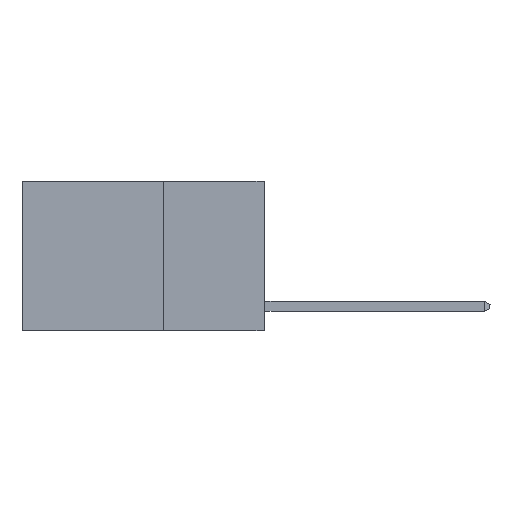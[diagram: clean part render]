
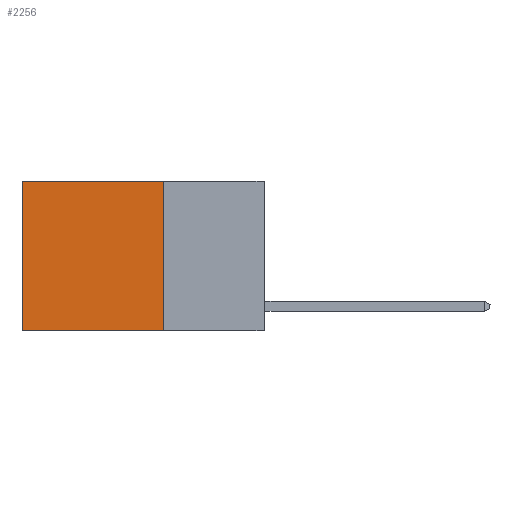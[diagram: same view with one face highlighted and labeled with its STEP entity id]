
A CAD part, left-side view. The second image highlights one B-rep face of the part: STEP entity #2256.
In plain terms, the highlighted planar face has unit normal (-1, 0, 0).
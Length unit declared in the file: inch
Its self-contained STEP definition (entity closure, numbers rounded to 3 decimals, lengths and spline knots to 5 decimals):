
#637 = LINE ( 'NONE', #5692, #11115 ) ;
#792 = ORIENTED_EDGE ( 'NONE', *, *, #3992, .T. ) ;
#971 = LINE ( 'NONE', #4453, #11431 ) ;
#973 = DIRECTION ( 'NONE',  ( 0., 1., 0. ) ) ;
#1138 = ORIENTED_EDGE ( 'NONE', *, *, #6979, .F. ) ;
#1245 = DIRECTION ( 'NONE',  ( 0., 1., 0. ) ) ;
#1276 = DIRECTION ( 'NONE',  ( 0., 0., -1. ) ) ;
#1631 = CARTESIAN_POINT ( 'NONE',  ( 0.2625, 0.6, 0. ) ) ;
#2208 = CARTESIAN_POINT ( 'NONE',  ( 0.2625, 0.6, -0.37 ) ) ;
#2256 = ADVANCED_FACE ( 'NONE', ( #8692 ), #10386, .F. ) ;
#2296 = CARTESIAN_POINT ( 'NONE',  ( 0.2625, 0.6, 0. ) ) ;
#2480 = AXIS2_PLACEMENT_3D ( 'NONE', #3639, #7596, #1276 ) ;
#2641 = CARTESIAN_POINT ( 'NONE',  ( 0.2625, 0.25, -0.37 ) ) ;
#3639 = CARTESIAN_POINT ( 'NONE',  ( 0.2625, 0.25, 0. ) ) ;
#3992 = EDGE_CURVE ( 'NONE', #9726, #4403, #6065, .T. ) ;
#4014 = DIRECTION ( 'NONE',  ( 0., 0., -1. ) ) ;
#4403 = VERTEX_POINT ( 'NONE', #2208 ) ;
#4453 = CARTESIAN_POINT ( 'NONE',  ( 0.2625, 0.25, 0. ) ) ;
#5239 = VECTOR ( 'NONE', #1245, 39.37008 ) ;
#5692 = CARTESIAN_POINT ( 'NONE',  ( 0.2625, 0.25, 0. ) ) ;
#5734 = DIRECTION ( 'NONE',  ( 0., 0., -1. ) ) ;
#5775 = VECTOR ( 'NONE', #4014, 39.37008 ) ;
#6065 = LINE ( 'NONE', #1631, #5775 ) ;
#6595 = CARTESIAN_POINT ( 'NONE',  ( 0.2625, 0.25, -0.37 ) ) ;
#6833 = ORIENTED_EDGE ( 'NONE', *, *, #9881, .F. ) ;
#6979 = EDGE_CURVE ( 'NONE', #9132, #4403, #12715, .T. ) ;
#7083 = EDGE_LOOP ( 'NONE', ( #792, #1138, #6833, #11844 ) ) ;
#7596 = DIRECTION ( 'NONE',  ( 1., 0., 0. ) ) ;
#7712 = VERTEX_POINT ( 'NONE', #7928 ) ;
#7928 = CARTESIAN_POINT ( 'NONE',  ( 0.2625, 0.25, 0. ) ) ;
#8692 = FACE_OUTER_BOUND ( 'NONE', #7083, .T. ) ;
#8842 = EDGE_CURVE ( 'NONE', #7712, #9726, #971, .T. ) ;
#9132 = VERTEX_POINT ( 'NONE', #2641 ) ;
#9726 = VERTEX_POINT ( 'NONE', #2296 ) ;
#9881 = EDGE_CURVE ( 'NONE', #7712, #9132, #637, .T. ) ;
#10386 = PLANE ( 'NONE',  #2480 ) ;
#11115 = VECTOR ( 'NONE', #5734, 39.37008 ) ;
#11431 = VECTOR ( 'NONE', #973, 39.37008 ) ;
#11844 = ORIENTED_EDGE ( 'NONE', *, *, #8842, .T. ) ;
#12715 = LINE ( 'NONE', #6595, #5239 ) ;
